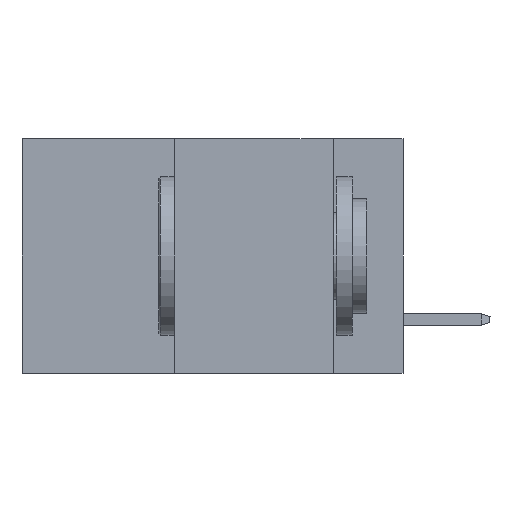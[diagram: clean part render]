
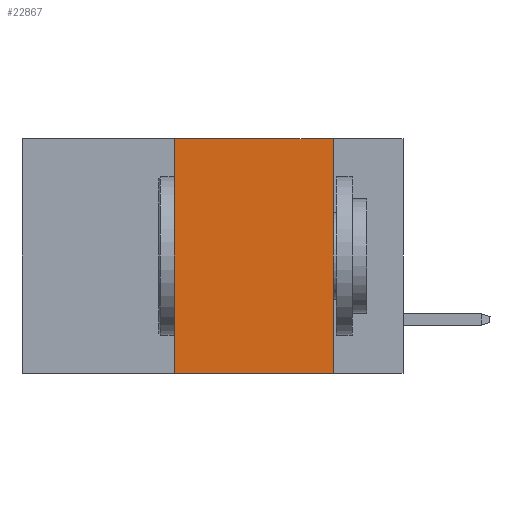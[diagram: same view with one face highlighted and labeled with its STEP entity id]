
A CAD part, left-side view. The second image highlights one B-rep face of the part: STEP entity #22867.
In plain terms, the highlighted planar face has unit normal (-1, 0, 0).
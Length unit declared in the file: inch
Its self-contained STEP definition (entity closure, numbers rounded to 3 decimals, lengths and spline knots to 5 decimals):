
#1990 = DIRECTION ( 'NONE',  ( 0., 0., -1. ) ) ;
#2127 = CARTESIAN_POINT ( 'NONE',  ( 0., 0.6, 0. ) ) ;
#2246 = DIRECTION ( 'NONE',  ( 0., 0., 1. ) ) ;
#2535 = AXIS2_PLACEMENT_3D ( 'NONE', #2127, #6476, #1990 ) ;
#2556 = VECTOR ( 'NONE', #2246, 39.37008 ) ;
#3021 = DIRECTION ( 'NONE',  ( 0., -1., 0. ) ) ;
#3035 = LINE ( 'NONE', #17327, #30381 ) ;
#3469 = ORIENTED_EDGE ( 'NONE', *, *, #23228, .F. ) ;
#3579 = CARTESIAN_POINT ( 'NONE',  ( 0., 0.11, -0.37 ) ) ;
#4559 = VERTEX_POINT ( 'NONE', #3579 ) ;
#5179 = CARTESIAN_POINT ( 'NONE',  ( 0., 0.11, 0. ) ) ;
#5561 = VERTEX_POINT ( 'NONE', #6756 ) ;
#6444 = CARTESIAN_POINT ( 'NONE',  ( 0., 0.36, 0. ) ) ;
#6469 = LINE ( 'NONE', #11127, #27377 ) ;
#6476 = DIRECTION ( 'NONE',  ( 1., 0., 0. ) ) ;
#6756 = CARTESIAN_POINT ( 'NONE',  ( 0., 0.36, -0.37 ) ) ;
#7013 = EDGE_CURVE ( 'NONE', #5561, #4559, #3035, .T. ) ;
#8621 = VERTEX_POINT ( 'NONE', #5179 ) ;
#8789 = DIRECTION ( 'NONE',  ( 0., 0., -1. ) ) ;
#8796 = PLANE ( 'NONE',  #2535 ) ;
#8987 = ORIENTED_EDGE ( 'NONE', *, *, #11780, .F. ) ;
#11127 = CARTESIAN_POINT ( 'NONE',  ( 0., 0.11, 0. ) ) ;
#11334 = CARTESIAN_POINT ( 'NONE',  ( 0., 0.36, 0. ) ) ;
#11780 = EDGE_CURVE ( 'NONE', #8621, #4559, #6469, .T. ) ;
#13175 = VECTOR ( 'NONE', #3021, 39.37008 ) ;
#14642 = EDGE_CURVE ( 'NONE', #18910, #8621, #19786, .T. ) ;
#17327 = CARTESIAN_POINT ( 'NONE',  ( 0., 0.6, -0.37 ) ) ;
#18542 = LINE ( 'NONE', #6444, #2556 ) ;
#18910 = VERTEX_POINT ( 'NONE', #11334 ) ;
#19786 = LINE ( 'NONE', #27046, #13175 ) ;
#19841 = ORIENTED_EDGE ( 'NONE', *, *, #7013, .T. ) ;
#22867 = ADVANCED_FACE ( 'NONE', ( #28170 ), #8796, .F. ) ;
#23228 = EDGE_CURVE ( 'NONE', #5561, #18910, #18542, .T. ) ;
#24176 = EDGE_LOOP ( 'NONE', ( #8987, #24431, #3469, #19841 ) ) ;
#24431 = ORIENTED_EDGE ( 'NONE', *, *, #14642, .F. ) ;
#24569 = DIRECTION ( 'NONE',  ( 0., -1., 0. ) ) ;
#27046 = CARTESIAN_POINT ( 'NONE',  ( 0., 0.6, 0. ) ) ;
#27377 = VECTOR ( 'NONE', #8789, 39.37008 ) ;
#28170 = FACE_OUTER_BOUND ( 'NONE', #24176, .T. ) ;
#30381 = VECTOR ( 'NONE', #24569, 39.37008 ) ;
